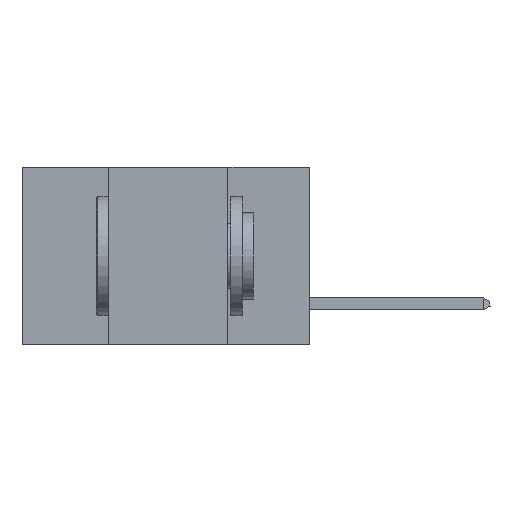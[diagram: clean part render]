
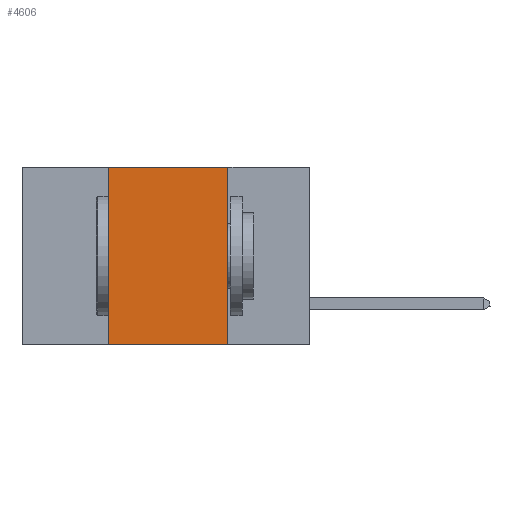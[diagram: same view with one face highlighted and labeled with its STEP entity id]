
A CAD part, left-side view. The second image highlights one B-rep face of the part: STEP entity #4606.
In plain terms, the highlighted planar face has unit normal (-1, 0, 0).
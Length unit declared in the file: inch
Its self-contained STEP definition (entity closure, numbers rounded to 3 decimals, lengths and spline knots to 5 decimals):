
#385 = EDGE_CURVE ( 'NONE', #40203, #2703, #20243, .T. ) ;
#1021 = CARTESIAN_POINT ( 'NONE',  ( 0., 0.42, 0. ) ) ;
#2318 = EDGE_CURVE ( 'NONE', #32669, #2703, #41477, .T. ) ;
#2479 = VERTEX_POINT ( 'NONE', #1021 ) ;
#2703 = VERTEX_POINT ( 'NONE', #32266 ) ;
#3626 = ORIENTED_EDGE ( 'NONE', *, *, #3770, .F. ) ;
#3770 = EDGE_CURVE ( 'NONE', #2479, #32669, #9533, .T. ) ;
#4606 = ADVANCED_FACE ( 'NONE', ( #29417 ), #8706, .F. ) ;
#4630 = CARTESIAN_POINT ( 'NONE',  ( 0., 0.6, -0.37 ) ) ;
#4744 = CARTESIAN_POINT ( 'NONE',  ( 0., 0.17, 0. ) ) ;
#6954 = CARTESIAN_POINT ( 'NONE',  ( 0., 0.42, -0.37 ) ) ;
#8706 = PLANE ( 'NONE',  #9508 ) ;
#9153 = DIRECTION ( 'NONE',  ( 1., 0., 0. ) ) ;
#9508 = AXIS2_PLACEMENT_3D ( 'NONE', #12217, #9153, #29534 ) ;
#9533 = LINE ( 'NONE', #11852, #17639 ) ;
#9948 = EDGE_CURVE ( 'NONE', #40203, #2479, #14274, .T. ) ;
#11736 = DIRECTION ( 'NONE',  ( 0., -1., 0. ) ) ;
#11852 = CARTESIAN_POINT ( 'NONE',  ( 0., 0.6, 0. ) ) ;
#12217 = CARTESIAN_POINT ( 'NONE',  ( 0., 0.6, 0. ) ) ;
#13618 = CARTESIAN_POINT ( 'NONE',  ( 0., 0.17, 0. ) ) ;
#14274 = LINE ( 'NONE', #25523, #40713 ) ;
#17639 = VECTOR ( 'NONE', #18905, 39.37008 ) ;
#18905 = DIRECTION ( 'NONE',  ( 0., -1., 0. ) ) ;
#19858 = VECTOR ( 'NONE', #30957, 39.37008 ) ;
#20243 = LINE ( 'NONE', #4630, #37549 ) ;
#25523 = CARTESIAN_POINT ( 'NONE',  ( 0., 0.42, 0. ) ) ;
#27776 = ORIENTED_EDGE ( 'NONE', *, *, #2318, .F. ) ;
#29417 = FACE_OUTER_BOUND ( 'NONE', #37601, .T. ) ;
#29534 = DIRECTION ( 'NONE',  ( 0., 0., -1. ) ) ;
#30957 = DIRECTION ( 'NONE',  ( 0., 0., -1. ) ) ;
#32266 = CARTESIAN_POINT ( 'NONE',  ( 0., 0.17, -0.37 ) ) ;
#32625 = ORIENTED_EDGE ( 'NONE', *, *, #385, .T. ) ;
#32669 = VERTEX_POINT ( 'NONE', #4744 ) ;
#37467 = ORIENTED_EDGE ( 'NONE', *, *, #9948, .F. ) ;
#37549 = VECTOR ( 'NONE', #11736, 39.37008 ) ;
#37601 = EDGE_LOOP ( 'NONE', ( #27776, #3626, #37467, #32625 ) ) ;
#39438 = DIRECTION ( 'NONE',  ( 0., 0., 1. ) ) ;
#40203 = VERTEX_POINT ( 'NONE', #6954 ) ;
#40713 = VECTOR ( 'NONE', #39438, 39.37008 ) ;
#41477 = LINE ( 'NONE', #13618, #19858 ) ;
